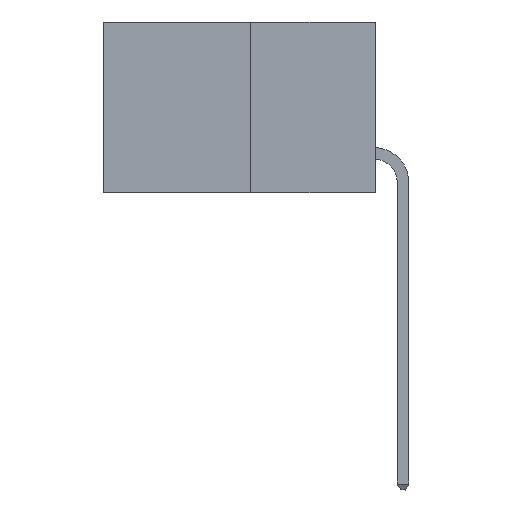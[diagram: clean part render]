
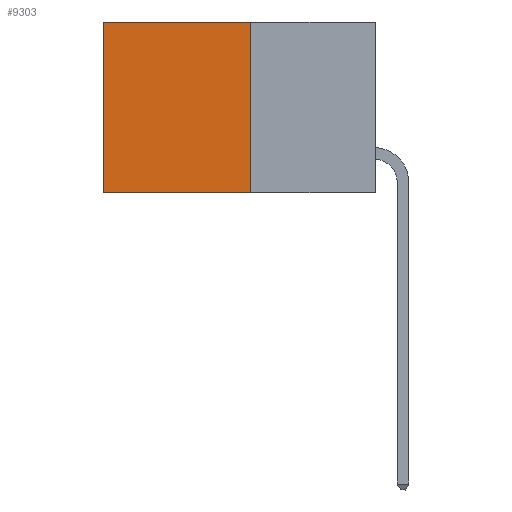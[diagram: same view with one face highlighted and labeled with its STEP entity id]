
A CAD part, left-side view. The second image highlights one B-rep face of the part: STEP entity #9303.
In plain terms, the highlighted planar face has unit normal (-1, 0, 0).
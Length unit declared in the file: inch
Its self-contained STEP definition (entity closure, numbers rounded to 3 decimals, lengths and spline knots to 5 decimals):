
#17 = EDGE_CURVE ( 'NONE', #930, #12510, #10235, .T. ) ;
#650 = CARTESIAN_POINT ( 'NONE',  ( 0.277, 0.59, 0. ) ) ;
#930 = VERTEX_POINT ( 'NONE', #650 ) ;
#1109 = ORIENTED_EDGE ( 'NONE', *, *, #13493, .F. ) ;
#2158 = AXIS2_PLACEMENT_3D ( 'NONE', #3018, #2999, #2958 ) ;
#2446 = EDGE_CURVE ( 'NONE', #8323, #11951, #2932, .T. ) ;
#2679 = VECTOR ( 'NONE', #9929, 39.37008 ) ;
#2916 = EDGE_LOOP ( 'NONE', ( #3762, #1109, #9793, #4455 ) ) ;
#2932 = LINE ( 'NONE', #11434, #13664 ) ;
#2958 = DIRECTION ( 'NONE',  ( 0., 0., -1. ) ) ;
#2999 = DIRECTION ( 'NONE',  ( 1., 0., 0. ) ) ;
#3016 = DIRECTION ( 'NONE',  ( 0., 1., 0. ) ) ;
#3018 = CARTESIAN_POINT ( 'NONE',  ( 0.277, 0.27, -0.37 ) ) ;
#3147 = PLANE ( 'NONE',  #2158 ) ;
#3762 = ORIENTED_EDGE ( 'NONE', *, *, #17, .T. ) ;
#4455 = ORIENTED_EDGE ( 'NONE', *, *, #5540, .T. ) ;
#4599 = CARTESIAN_POINT ( 'NONE',  ( 0.277, 0.59, -0.37 ) ) ;
#5540 = EDGE_CURVE ( 'NONE', #8323, #930, #8738, .T. ) ;
#5941 = CARTESIAN_POINT ( 'NONE',  ( 0.277, 0.27, -0.37 ) ) ;
#6206 = LINE ( 'NONE', #12712, #8661 ) ;
#6296 = CARTESIAN_POINT ( 'NONE',  ( 0.277, 0.27, 0. ) ) ;
#6701 = CARTESIAN_POINT ( 'NONE',  ( 0.277, 0.59, -0.37 ) ) ;
#8323 = VERTEX_POINT ( 'NONE', #13099 ) ;
#8661 = VECTOR ( 'NONE', #3016, 39.37008 ) ;
#8738 = LINE ( 'NONE', #6296, #2679 ) ;
#9303 = ADVANCED_FACE ( 'NONE', ( #10985 ), #3147, .F. ) ;
#9492 = DIRECTION ( 'NONE',  ( 0., 0., -1. ) ) ;
#9793 = ORIENTED_EDGE ( 'NONE', *, *, #2446, .F. ) ;
#9929 = DIRECTION ( 'NONE',  ( 0., 1., 0. ) ) ;
#10235 = LINE ( 'NONE', #6701, #13075 ) ;
#10399 = DIRECTION ( 'NONE',  ( 0., 0., -1. ) ) ;
#10985 = FACE_OUTER_BOUND ( 'NONE', #2916, .T. ) ;
#11434 = CARTESIAN_POINT ( 'NONE',  ( 0.277, 0.27, -0.37 ) ) ;
#11951 = VERTEX_POINT ( 'NONE', #5941 ) ;
#12510 = VERTEX_POINT ( 'NONE', #4599 ) ;
#12712 = CARTESIAN_POINT ( 'NONE',  ( 0.277, 0.27, -0.37 ) ) ;
#13075 = VECTOR ( 'NONE', #9492, 39.37008 ) ;
#13099 = CARTESIAN_POINT ( 'NONE',  ( 0.277, 0.27, 0. ) ) ;
#13493 = EDGE_CURVE ( 'NONE', #11951, #12510, #6206, .T. ) ;
#13664 = VECTOR ( 'NONE', #10399, 39.37008 ) ;
